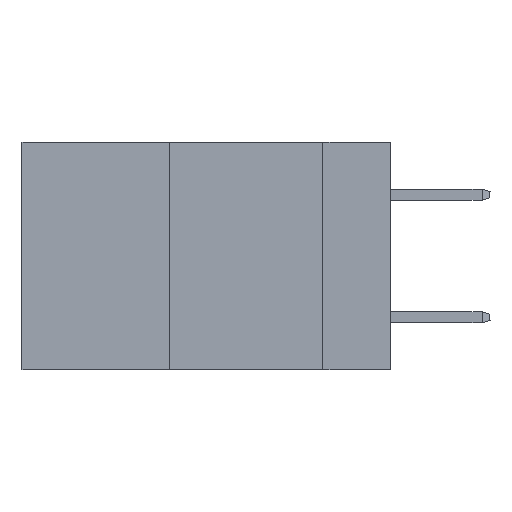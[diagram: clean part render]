
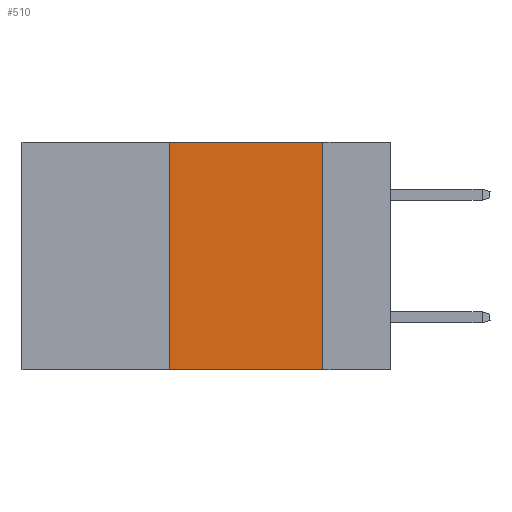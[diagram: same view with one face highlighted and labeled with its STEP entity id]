
A CAD part, left-side view. The second image highlights one B-rep face of the part: STEP entity #510.
In plain terms, the highlighted planar face has unit normal (-1, 0, 0).
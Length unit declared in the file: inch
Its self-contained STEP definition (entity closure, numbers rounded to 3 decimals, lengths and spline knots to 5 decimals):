
#119 = DIRECTION ( 'NONE',  ( 1., 0., 0. ) ) ;
#161 = LINE ( 'NONE', #314, #8126 ) ;
#314 = CARTESIAN_POINT ( 'NONE',  ( 0., 0.6, 0. ) ) ;
#507 = ORIENTED_EDGE ( 'NONE', *, *, #9833, .T. ) ;
#510 = ADVANCED_FACE ( 'NONE', ( #4893 ), #7326, .F. ) ;
#985 = CARTESIAN_POINT ( 'NONE',  ( 0., 0.6, 0. ) ) ;
#1184 = AXIS2_PLACEMENT_3D ( 'NONE', #985, #119, #5083 ) ;
#2137 = VECTOR ( 'NONE', #10561, 39.37008 ) ;
#2400 = CARTESIAN_POINT ( 'NONE',  ( 0., 0.11, 0. ) ) ;
#2784 = VERTEX_POINT ( 'NONE', #11009 ) ;
#3155 = EDGE_CURVE ( 'NONE', #2784, #12156, #161, .T. ) ;
#3441 = VECTOR ( 'NONE', #5397, 39.37008 ) ;
#4139 = LINE ( 'NONE', #10695, #2137 ) ;
#4169 = VECTOR ( 'NONE', #6505, 39.37008 ) ;
#4176 = ORIENTED_EDGE ( 'NONE', *, *, #8918, .F. ) ;
#4506 = CARTESIAN_POINT ( 'NONE',  ( 0., 0.36, 0. ) ) ;
#4893 = FACE_OUTER_BOUND ( 'NONE', #7555, .T. ) ;
#5083 = DIRECTION ( 'NONE',  ( 0., 0., -1. ) ) ;
#5397 = DIRECTION ( 'NONE',  ( 0., 0., -1. ) ) ;
#5420 = VERTEX_POINT ( 'NONE', #6596 ) ;
#6475 = EDGE_CURVE ( 'NONE', #12156, #6522, #9047, .T. ) ;
#6505 = DIRECTION ( 'NONE',  ( 0., 0., 1. ) ) ;
#6522 = VERTEX_POINT ( 'NONE', #7165 ) ;
#6596 = CARTESIAN_POINT ( 'NONE',  ( 0., 0.36, -0.37 ) ) ;
#7032 = ORIENTED_EDGE ( 'NONE', *, *, #3155, .F. ) ;
#7165 = CARTESIAN_POINT ( 'NONE',  ( 0., 0.11, -0.37 ) ) ;
#7326 = PLANE ( 'NONE',  #1184 ) ;
#7555 = EDGE_LOOP ( 'NONE', ( #11994, #7032, #4176, #507 ) ) ;
#8126 = VECTOR ( 'NONE', #9236, 39.37008 ) ;
#8918 = EDGE_CURVE ( 'NONE', #5420, #2784, #11949, .T. ) ;
#9047 = LINE ( 'NONE', #10515, #3441 ) ;
#9236 = DIRECTION ( 'NONE',  ( 0., -1., 0. ) ) ;
#9833 = EDGE_CURVE ( 'NONE', #5420, #6522, #4139, .T. ) ;
#10515 = CARTESIAN_POINT ( 'NONE',  ( 0., 0.11, 0. ) ) ;
#10561 = DIRECTION ( 'NONE',  ( 0., -1., 0. ) ) ;
#10695 = CARTESIAN_POINT ( 'NONE',  ( 0., 0.6, -0.37 ) ) ;
#11009 = CARTESIAN_POINT ( 'NONE',  ( 0., 0.36, 0. ) ) ;
#11949 = LINE ( 'NONE', #4506, #4169 ) ;
#11994 = ORIENTED_EDGE ( 'NONE', *, *, #6475, .F. ) ;
#12156 = VERTEX_POINT ( 'NONE', #2400 ) ;
